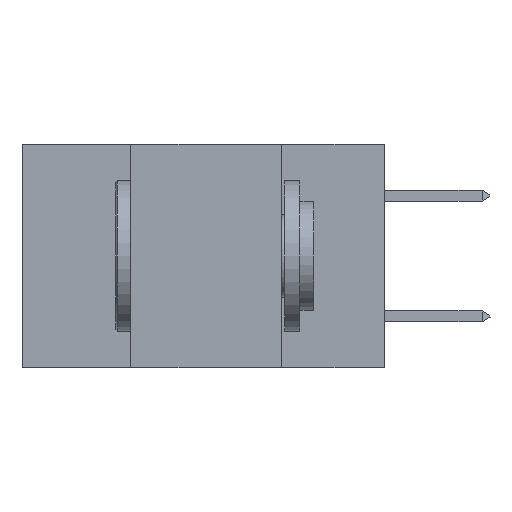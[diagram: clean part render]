
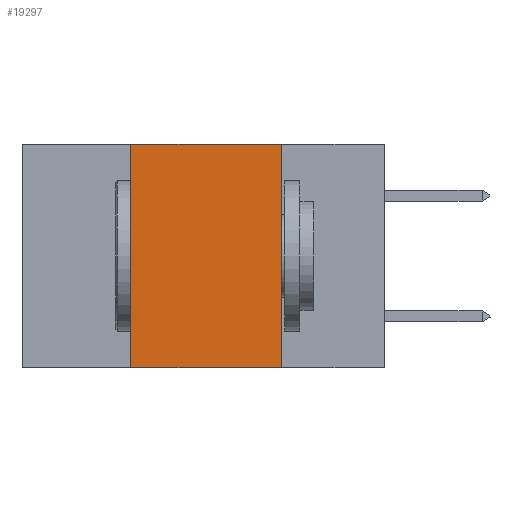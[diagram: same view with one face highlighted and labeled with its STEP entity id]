
A CAD part, left-side view. The second image highlights one B-rep face of the part: STEP entity #19297.
In plain terms, the highlighted planar face has unit normal (-1, 0, 0).
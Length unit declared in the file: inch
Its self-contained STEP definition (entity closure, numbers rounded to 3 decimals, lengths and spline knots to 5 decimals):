
#1808 = EDGE_LOOP ( 'NONE', ( #12547, #10175, #10877, #8210 ) ) ;
#1951 = EDGE_CURVE ( 'NONE', #6450, #12063, #6099, .T. ) ;
#2255 = CARTESIAN_POINT ( 'NONE',  ( 0., 0.6, 0. ) ) ;
#2387 = VERTEX_POINT ( 'NONE', #2828 ) ;
#2538 = DIRECTION ( 'NONE',  ( 0., -1., 0. ) ) ;
#2767 = DIRECTION ( 'NONE',  ( 1., 0., 0. ) ) ;
#2828 = CARTESIAN_POINT ( 'NONE',  ( 0., 0.17, 0. ) ) ;
#3037 = LINE ( 'NONE', #2255, #10843 ) ;
#3932 = VECTOR ( 'NONE', #12688, 39.37008 ) ;
#4017 = VERTEX_POINT ( 'NONE', #17920 ) ;
#4291 = CARTESIAN_POINT ( 'NONE',  ( 0., 0.42, 0. ) ) ;
#4494 = PLANE ( 'NONE',  #18854 ) ;
#5106 = CARTESIAN_POINT ( 'NONE',  ( 0., 0.42, -0.37 ) ) ;
#5859 = DIRECTION ( 'NONE',  ( 0., 0., -1. ) ) ;
#6089 = CARTESIAN_POINT ( 'NONE',  ( 0., 0.6, 0. ) ) ;
#6099 = LINE ( 'NONE', #15380, #13657 ) ;
#6450 = VERTEX_POINT ( 'NONE', #5106 ) ;
#8108 = LINE ( 'NONE', #11233, #3932 ) ;
#8210 = ORIENTED_EDGE ( 'NONE', *, *, #13641, .T. ) ;
#10175 = ORIENTED_EDGE ( 'NONE', *, *, #12090, .F. ) ;
#10514 = LINE ( 'NONE', #13624, #19794 ) ;
#10633 = FACE_OUTER_BOUND ( 'NONE', #1808, .T. ) ;
#10711 = DIRECTION ( 'NONE',  ( 0., 0., 1. ) ) ;
#10843 = VECTOR ( 'NONE', #2538, 39.37008 ) ;
#10877 = ORIENTED_EDGE ( 'NONE', *, *, #1951, .F. ) ;
#11233 = CARTESIAN_POINT ( 'NONE',  ( 0., 0.6, -0.37 ) ) ;
#12063 = VERTEX_POINT ( 'NONE', #4291 ) ;
#12090 = EDGE_CURVE ( 'NONE', #12063, #2387, #3037, .T. ) ;
#12547 = ORIENTED_EDGE ( 'NONE', *, *, #13994, .F. ) ;
#12688 = DIRECTION ( 'NONE',  ( 0., -1., 0. ) ) ;
#13624 = CARTESIAN_POINT ( 'NONE',  ( 0., 0.17, 0. ) ) ;
#13641 = EDGE_CURVE ( 'NONE', #6450, #4017, #8108, .T. ) ;
#13657 = VECTOR ( 'NONE', #10711, 39.37008 ) ;
#13714 = DIRECTION ( 'NONE',  ( 0., 0., -1. ) ) ;
#13994 = EDGE_CURVE ( 'NONE', #2387, #4017, #10514, .T. ) ;
#15380 = CARTESIAN_POINT ( 'NONE',  ( 0., 0.42, 0. ) ) ;
#17920 = CARTESIAN_POINT ( 'NONE',  ( 0., 0.17, -0.37 ) ) ;
#18854 = AXIS2_PLACEMENT_3D ( 'NONE', #6089, #2767, #13714 ) ;
#19297 = ADVANCED_FACE ( 'NONE', ( #10633 ), #4494, .F. ) ;
#19794 = VECTOR ( 'NONE', #5859, 39.37008 ) ;
